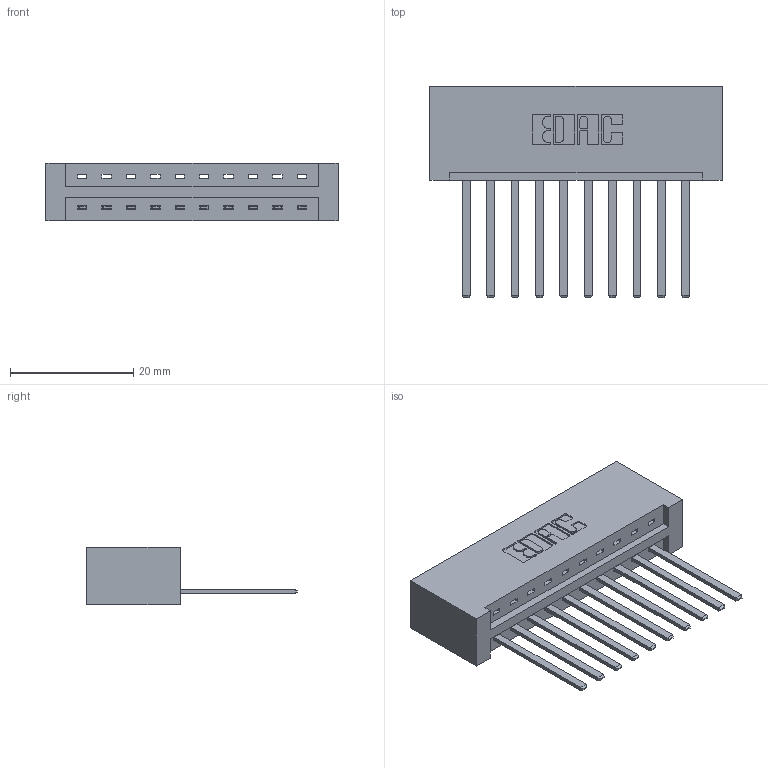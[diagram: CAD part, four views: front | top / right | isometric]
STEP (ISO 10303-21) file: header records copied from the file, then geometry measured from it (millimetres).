
FILE_DESCRIPTION (( 'STEP AP203' ), '1' );
FILE_NAME ('387-010-544-101.STEP', '2019-10-02T11:37:50', ( '' ), ( '' ), 'SwSTEP 2.0', 'SolidWorks 2016', '' );
FILE_SCHEMA (( 'CONFIG_CONTROL_DESIGN' ));
Length unit declared in the file: inch
Products named in the file (3): 387-010-544-101; 345-292-001_345-293-144; 337 Part_No Mounting Lugs
Assembly tree (11 placements, depth 2):
  387-010-544-101
    337 Part_No Mounting Lugs
    345-292-001_345-293-144  x10
Bounding box: 47.5 x 34.3 x 9.4 mm (x, y, z)
Volume: 5390.7 mm3; surface area: 5755.3 mm2
Topology: 11 solids, 11 shells, 666 faces, 1987 edges, 1310 vertices
Faces by surface type: plane 486, cylinder 180
Entity records: 11111 total; most frequent: CARTESIAN_POINT 1940, ORIENTED_EDGE 1886, DIRECTION 1687, EDGE_CURVE 943, LINE 827, VECTOR 827, VERTEX_POINT 626, AXIS2_PLACEMENT_3D 430
